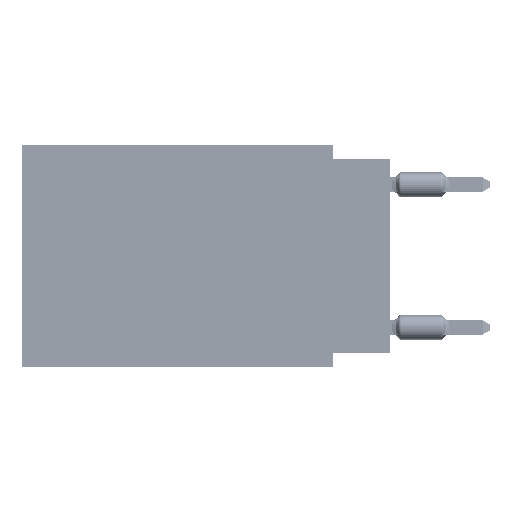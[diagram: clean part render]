
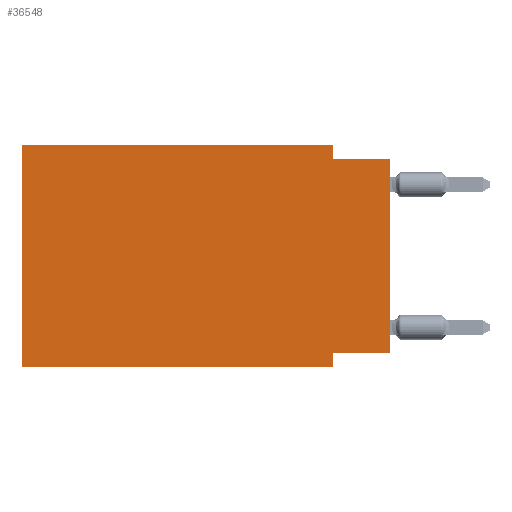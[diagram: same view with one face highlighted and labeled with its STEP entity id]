
A CAD part, left-side view. The second image highlights one B-rep face of the part: STEP entity #36548.
In plain terms, the highlighted planar face has unit normal (-1, 0, 0).
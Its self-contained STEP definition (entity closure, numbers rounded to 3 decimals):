
#58 = VECTOR ( 'NONE', #43249, 1000. ) ;
#1188 = CARTESIAN_POINT ( 'NONE',  ( 0., 16.383, 0. ) ) ;
#1514 = EDGE_CURVE ( 'NONE', #22393, #42130, #28441, .T. ) ;
#1518 = AXIS2_PLACEMENT_3D ( 'NONE', #1188, #17966, #54769 ) ;
#2822 = CARTESIAN_POINT ( 'NONE',  ( 0., 0., -9.271 ) ) ;
#3119 = VECTOR ( 'NONE', #45535, 1000. ) ;
#4356 = ORIENTED_EDGE ( 'NONE', *, *, #28832, .F. ) ;
#5724 = ORIENTED_EDGE ( 'NONE', *, *, #55598, .T. ) ;
#6275 = ORIENTED_EDGE ( 'NONE', *, *, #65247, .T. ) ;
#7982 = CARTESIAN_POINT ( 'NONE',  ( 0., 16.383, 0. ) ) ;
#8388 = VERTEX_POINT ( 'NONE', #11555 ) ;
#8935 = ORIENTED_EDGE ( 'NONE', *, *, #1514, .F. ) ;
#9573 = CARTESIAN_POINT ( 'NONE',  ( 0., 16.383, -9.906 ) ) ;
#10124 = VECTOR ( 'NONE', #35237, 1000. ) ;
#10164 = VECTOR ( 'NONE', #26535, 1000. ) ;
#10692 = LINE ( 'NONE', #69172, #58 ) ;
#11555 = CARTESIAN_POINT ( 'NONE',  ( 0., 0., -9.271 ) ) ;
#11692 = PLANE ( 'NONE',  #1518 ) ;
#12191 = ORIENTED_EDGE ( 'NONE', *, *, #35036, .F. ) ;
#12717 = EDGE_CURVE ( 'NONE', #42130, #57679, #61214, .T. ) ;
#17966 = DIRECTION ( 'NONE',  ( 1., 0., 0. ) ) ;
#18055 = LINE ( 'NONE', #58829, #25527 ) ;
#18293 = CARTESIAN_POINT ( 'NONE',  ( 0., 2.54, -9.906 ) ) ;
#22393 = VERTEX_POINT ( 'NONE', #9573 ) ;
#23213 = FACE_OUTER_BOUND ( 'NONE', #60979, .T. ) ;
#23687 = VECTOR ( 'NONE', #66583, 1000. ) ;
#24175 = LINE ( 'NONE', #2822, #3119 ) ;
#24534 = CARTESIAN_POINT ( 'NONE',  ( 0., 2.54, 0. ) ) ;
#25262 = CARTESIAN_POINT ( 'NONE',  ( 0., 2.54, 0. ) ) ;
#25527 = VECTOR ( 'NONE', #31871, 1000. ) ;
#26187 = EDGE_CURVE ( 'NONE', #8388, #47459, #24175, .T. ) ;
#26535 = DIRECTION ( 'NONE',  ( 0., 0., -1. ) ) ;
#28441 = LINE ( 'NONE', #44553, #52437 ) ;
#28832 = EDGE_CURVE ( 'NONE', #56207, #48344, #18055, .T. ) ;
#29277 = LINE ( 'NONE', #50659, #10124 ) ;
#29337 = DIRECTION ( 'NONE',  ( 0., -1., 0. ) ) ;
#31871 = DIRECTION ( 'NONE',  ( 0., -1., 0. ) ) ;
#34049 = DIRECTION ( 'NONE',  ( 0., 0., 1. ) ) ;
#35036 = EDGE_CURVE ( 'NONE', #57679, #56207, #45207, .T. ) ;
#35237 = DIRECTION ( 'NONE',  ( 0., -1., 0. ) ) ;
#36548 = ADVANCED_FACE ( 'NONE', ( #23213 ), #11692, .F. ) ;
#37908 = CARTESIAN_POINT ( 'NONE',  ( 0., 0., -0.635 ) ) ;
#38825 = EDGE_CURVE ( 'NONE', #47459, #67206, #53150, .T. ) ;
#39051 = ORIENTED_EDGE ( 'NONE', *, *, #26187, .F. ) ;
#42130 = VERTEX_POINT ( 'NONE', #65340 ) ;
#43249 = DIRECTION ( 'NONE',  ( 0., 0., 1. ) ) ;
#44199 = CARTESIAN_POINT ( 'NONE',  ( 0., 2.54, -0.635 ) ) ;
#44553 = CARTESIAN_POINT ( 'NONE',  ( 0., 16.383, 0. ) ) ;
#45207 = LINE ( 'NONE', #24534, #23687 ) ;
#45535 = DIRECTION ( 'NONE',  ( 0., 1., 0. ) ) ;
#47459 = VERTEX_POINT ( 'NONE', #65461 ) ;
#48344 = VERTEX_POINT ( 'NONE', #37908 ) ;
#50659 = CARTESIAN_POINT ( 'NONE',  ( 0., 16.383, -9.906 ) ) ;
#52437 = VECTOR ( 'NONE', #34049, 1000. ) ;
#53150 = LINE ( 'NONE', #58063, #10164 ) ;
#54159 = ORIENTED_EDGE ( 'NONE', *, *, #38825, .F. ) ;
#54769 = DIRECTION ( 'NONE',  ( 0., 0., -1. ) ) ;
#55598 = EDGE_CURVE ( 'NONE', #8388, #48344, #10692, .T. ) ;
#56207 = VERTEX_POINT ( 'NONE', #44199 ) ;
#57153 = ORIENTED_EDGE ( 'NONE', *, *, #12717, .F. ) ;
#57679 = VERTEX_POINT ( 'NONE', #25262 ) ;
#58063 = CARTESIAN_POINT ( 'NONE',  ( 0., 2.54, -9.906 ) ) ;
#58829 = CARTESIAN_POINT ( 'NONE',  ( 0., 0., -0.635 ) ) ;
#60979 = EDGE_LOOP ( 'NONE', ( #5724, #4356, #12191, #57153, #8935, #6275, #54159, #39051 ) ) ;
#61214 = LINE ( 'NONE', #7982, #65084 ) ;
#65084 = VECTOR ( 'NONE', #29337, 1000. ) ;
#65247 = EDGE_CURVE ( 'NONE', #22393, #67206, #29277, .T. ) ;
#65340 = CARTESIAN_POINT ( 'NONE',  ( 0., 16.383, 0. ) ) ;
#65461 = CARTESIAN_POINT ( 'NONE',  ( 0., 2.54, -9.271 ) ) ;
#66583 = DIRECTION ( 'NONE',  ( 0., 0., -1. ) ) ;
#67206 = VERTEX_POINT ( 'NONE', #18293 ) ;
#69172 = CARTESIAN_POINT ( 'NONE',  ( 0., 0., 0. ) ) ;
